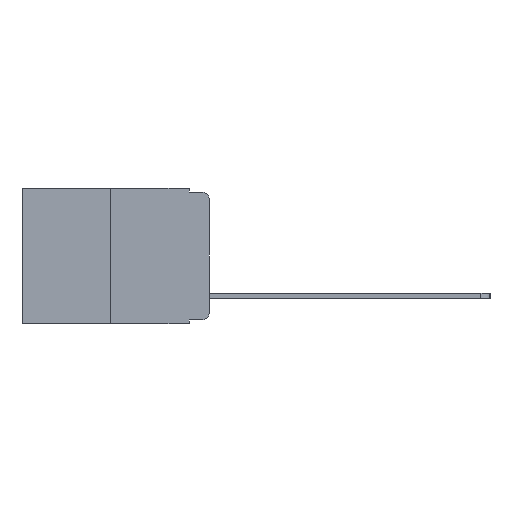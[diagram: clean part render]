
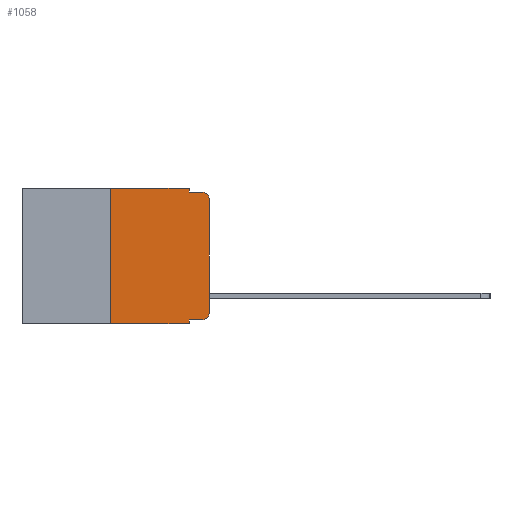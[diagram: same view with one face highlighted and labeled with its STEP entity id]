
A CAD part, left-side view. The second image highlights one B-rep face of the part: STEP entity #1058.
In plain terms, the highlighted planar face has unit normal (-1, 0, 0).
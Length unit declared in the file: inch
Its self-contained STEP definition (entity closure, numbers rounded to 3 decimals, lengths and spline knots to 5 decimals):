
#313 = ORIENTED_EDGE ( 'NONE', *, *, #905, .T. ) ;
#339 = VERTEX_POINT ( 'NONE', #10695 ) ;
#411 = CARTESIAN_POINT ( 'NONE',  ( 0., 0.02, -0.01 ) ) ;
#434 = EDGE_CURVE ( 'NONE', #3443, #3720, #6306, .T. ) ;
#482 = CARTESIAN_POINT ( 'NONE',  ( 0., 0., 0. ) ) ;
#483 = VERTEX_POINT ( 'NONE', #3268 ) ;
#509 = CARTESIAN_POINT ( 'NONE',  ( 0., 0.473, 0. ) ) ;
#609 = VECTOR ( 'NONE', #6557, 39.37008 ) ;
#670 = ORIENTED_EDGE ( 'NONE', *, *, #3842, .F. ) ;
#905 = EDGE_CURVE ( 'NONE', #10300, #8481, #7927, .T. ) ;
#916 = VECTOR ( 'NONE', #3992, 39.37008 ) ;
#1058 = ADVANCED_FACE ( 'NONE', ( #1577 ), #2266, .F. ) ;
#1092 = CARTESIAN_POINT ( 'NONE',  ( 0., 0.25, -0.343 ) ) ;
#1149 = EDGE_CURVE ( 'NONE', #1864, #3443, #3630, .T. ) ;
#1249 = AXIS2_PLACEMENT_3D ( 'NONE', #1496, #1356, #1380 ) ;
#1356 = DIRECTION ( 'NONE',  ( -1., 0., 0. ) ) ;
#1380 = DIRECTION ( 'NONE',  ( 0., 0., -1. ) ) ;
#1496 = CARTESIAN_POINT ( 'NONE',  ( 0., 0.02, -0.313 ) ) ;
#1577 = FACE_OUTER_BOUND ( 'NONE', #9239, .T. ) ;
#1631 = VERTEX_POINT ( 'NONE', #411 ) ;
#1864 = VERTEX_POINT ( 'NONE', #2790 ) ;
#1981 = CARTESIAN_POINT ( 'NONE',  ( 0., 0.051, 0. ) ) ;
#2229 = LINE ( 'NONE', #482, #11237 ) ;
#2266 = PLANE ( 'NONE',  #9670 ) ;
#2405 = VERTEX_POINT ( 'NONE', #4438 ) ;
#2501 = EDGE_CURVE ( 'NONE', #1864, #8481, #10473, .T. ) ;
#2544 = DIRECTION ( 'NONE',  ( 0., 0., 1. ) ) ;
#2609 = CARTESIAN_POINT ( 'NONE',  ( 0., 0.051, 0. ) ) ;
#2790 = CARTESIAN_POINT ( 'NONE',  ( 0., 0.051, -0.333 ) ) ;
#3268 = CARTESIAN_POINT ( 'NONE',  ( 0., 0.25, 0. ) ) ;
#3350 = CARTESIAN_POINT ( 'NONE',  ( 0., 0.25, 0. ) ) ;
#3443 = VERTEX_POINT ( 'NONE', #7216 ) ;
#3629 = DIRECTION ( 'NONE',  ( 1., 0., 0. ) ) ;
#3630 = LINE ( 'NONE', #5526, #609 ) ;
#3669 = ORIENTED_EDGE ( 'NONE', *, *, #1149, .T. ) ;
#3720 = VERTEX_POINT ( 'NONE', #6238 ) ;
#3842 = EDGE_CURVE ( 'NONE', #10300, #483, #4707, .T. ) ;
#3992 = DIRECTION ( 'NONE',  ( 0., 0., -1. ) ) ;
#4265 = ORIENTED_EDGE ( 'NONE', *, *, #434, .T. ) ;
#4438 = CARTESIAN_POINT ( 'NONE',  ( 0., 0.051, 0. ) ) ;
#4706 = VERTEX_POINT ( 'NONE', #11119 ) ;
#4707 = LINE ( 'NONE', #3350, #11172 ) ;
#4951 = ORIENTED_EDGE ( 'NONE', *, *, #5644, .F. ) ;
#5049 = EDGE_CURVE ( 'NONE', #2405, #4706, #11490, .T. ) ;
#5239 = ORIENTED_EDGE ( 'NONE', *, *, #5049, .F. ) ;
#5368 = VECTOR ( 'NONE', #7203, 39.37008 ) ;
#5526 = CARTESIAN_POINT ( 'NONE',  ( 0., 0.051, -0.333 ) ) ;
#5531 = DIRECTION ( 'NONE',  ( -1., 0., 0. ) ) ;
#5616 = VECTOR ( 'NONE', #6122, 39.37008 ) ;
#5644 = EDGE_CURVE ( 'NONE', #4706, #1631, #7689, .T. ) ;
#5966 = CARTESIAN_POINT ( 'NONE',  ( 0., 0.051, -0.01 ) ) ;
#6088 = ORIENTED_EDGE ( 'NONE', *, *, #2501, .F. ) ;
#6122 = DIRECTION ( 'NONE',  ( 0., -1., 0. ) ) ;
#6238 = CARTESIAN_POINT ( 'NONE',  ( 0., 0., -0.313 ) ) ;
#6306 = CIRCLE ( 'NONE', #1249, 0.02 ) ;
#6557 = DIRECTION ( 'NONE',  ( 0., -1., 0. ) ) ;
#6595 = CIRCLE ( 'NONE', #7682, 0.02 ) ;
#6754 = CARTESIAN_POINT ( 'NONE',  ( 0., 0.473, 0. ) ) ;
#6818 = EDGE_CURVE ( 'NONE', #3720, #339, #2229, .T. ) ;
#7203 = DIRECTION ( 'NONE',  ( 0., -1., 0. ) ) ;
#7216 = CARTESIAN_POINT ( 'NONE',  ( 0., 0.02, -0.333 ) ) ;
#7263 = LINE ( 'NONE', #6754, #9247 ) ;
#7292 = ORIENTED_EDGE ( 'NONE', *, *, #7561, .F. ) ;
#7414 = EDGE_CURVE ( 'NONE', #339, #1631, #6595, .T. ) ;
#7561 = EDGE_CURVE ( 'NONE', #483, #2405, #7263, .T. ) ;
#7682 = AXIS2_PLACEMENT_3D ( 'NONE', #10591, #5531, #11358 ) ;
#7689 = LINE ( 'NONE', #5966, #5368 ) ;
#7927 = LINE ( 'NONE', #9821, #5616 ) ;
#8481 = VERTEX_POINT ( 'NONE', #10634 ) ;
#8511 = DIRECTION ( 'NONE',  ( 0., -1., 0. ) ) ;
#8704 = DIRECTION ( 'NONE',  ( 0., 0., -1. ) ) ;
#9239 = EDGE_LOOP ( 'NONE', ( #9279, #9658, #4951, #5239, #7292, #670, #313, #6088, #3669, #4265 ) ) ;
#9247 = VECTOR ( 'NONE', #8511, 39.37008 ) ;
#9279 = ORIENTED_EDGE ( 'NONE', *, *, #6818, .T. ) ;
#9326 = DIRECTION ( 'NONE',  ( 0., 0., 1. ) ) ;
#9418 = VECTOR ( 'NONE', #8704, 39.37008 ) ;
#9658 = ORIENTED_EDGE ( 'NONE', *, *, #7414, .T. ) ;
#9670 = AXIS2_PLACEMENT_3D ( 'NONE', #509, #3629, #10706 ) ;
#9821 = CARTESIAN_POINT ( 'NONE',  ( 0., 0.473, -0.343 ) ) ;
#10300 = VERTEX_POINT ( 'NONE', #1092 ) ;
#10473 = LINE ( 'NONE', #2609, #916 ) ;
#10591 = CARTESIAN_POINT ( 'NONE',  ( 0., 0.02, -0.03 ) ) ;
#10634 = CARTESIAN_POINT ( 'NONE',  ( 0., 0.051, -0.343 ) ) ;
#10695 = CARTESIAN_POINT ( 'NONE',  ( 0., 0., -0.03 ) ) ;
#10706 = DIRECTION ( 'NONE',  ( 0., 0., -1. ) ) ;
#11119 = CARTESIAN_POINT ( 'NONE',  ( 0., 0.051, -0.01 ) ) ;
#11172 = VECTOR ( 'NONE', #9326, 39.37008 ) ;
#11237 = VECTOR ( 'NONE', #2544, 39.37008 ) ;
#11358 = DIRECTION ( 'NONE',  ( 0., 0., -1. ) ) ;
#11490 = LINE ( 'NONE', #1981, #9418 ) ;
